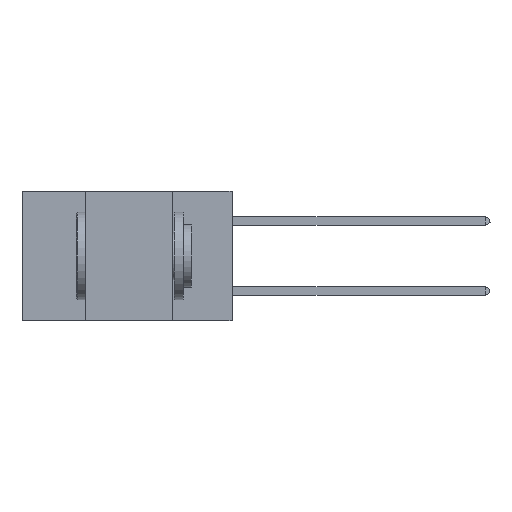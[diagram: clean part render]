
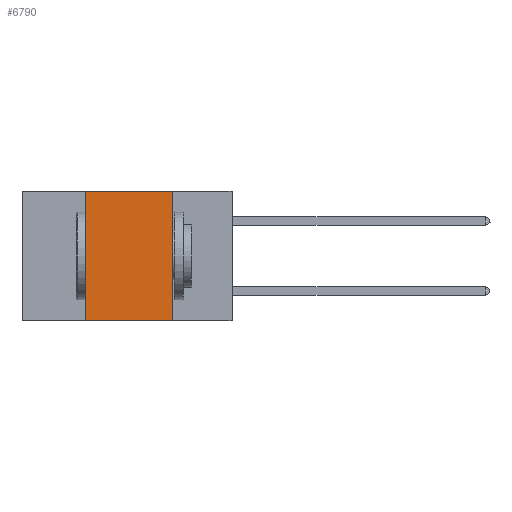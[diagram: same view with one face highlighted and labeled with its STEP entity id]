
A CAD part, left-side view. The second image highlights one B-rep face of the part: STEP entity #6790.
In plain terms, the highlighted planar face has unit normal (-1, 0, 0).
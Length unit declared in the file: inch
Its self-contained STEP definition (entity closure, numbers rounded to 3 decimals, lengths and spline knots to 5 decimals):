
#11 = DIRECTION ( 'NONE',  ( 0., -1., 0. ) ) ;
#507 = ORIENTED_EDGE ( 'NONE', *, *, #2817, .T. ) ;
#767 = CARTESIAN_POINT ( 'NONE',  ( 0., 0.6, 0. ) ) ;
#942 = VECTOR ( 'NONE', #11, 39.37008 ) ;
#2387 = CARTESIAN_POINT ( 'NONE',  ( 0., 0.6, 0. ) ) ;
#2694 = VERTEX_POINT ( 'NONE', #7048 ) ;
#2817 = EDGE_CURVE ( 'NONE', #7600, #11250, #10551, .T. ) ;
#3589 = CARTESIAN_POINT ( 'NONE',  ( 0., 0.6, -0.37 ) ) ;
#4266 = EDGE_CURVE ( 'NONE', #2694, #7081, #11045, .T. ) ;
#4537 = LINE ( 'NONE', #8906, #6108 ) ;
#4671 = EDGE_LOOP ( 'NONE', ( #9125, #9082, #5598, #507 ) ) ;
#4941 = LINE ( 'NONE', #5986, #10848 ) ;
#5598 = ORIENTED_EDGE ( 'NONE', *, *, #10435, .F. ) ;
#5986 = CARTESIAN_POINT ( 'NONE',  ( 0., 0.42, 0. ) ) ;
#6108 = VECTOR ( 'NONE', #8002, 39.37008 ) ;
#6155 = DIRECTION ( 'NONE',  ( 0., -1., 0. ) ) ;
#6216 = PLANE ( 'NONE',  #10685 ) ;
#6446 = CARTESIAN_POINT ( 'NONE',  ( 0., 0.17, 0. ) ) ;
#6533 = EDGE_CURVE ( 'NONE', #7081, #11250, #4537, .T. ) ;
#6790 = ADVANCED_FACE ( 'NONE', ( #10451 ), #6216, .F. ) ;
#7048 = CARTESIAN_POINT ( 'NONE',  ( 0., 0.42, 0. ) ) ;
#7081 = VERTEX_POINT ( 'NONE', #6446 ) ;
#7139 = DIRECTION ( 'NONE',  ( 1., 0., 0. ) ) ;
#7442 = VECTOR ( 'NONE', #6155, 39.37008 ) ;
#7600 = VERTEX_POINT ( 'NONE', #11287 ) ;
#8002 = DIRECTION ( 'NONE',  ( 0., 0., -1. ) ) ;
#8051 = DIRECTION ( 'NONE',  ( 0., 0., -1. ) ) ;
#8906 = CARTESIAN_POINT ( 'NONE',  ( 0., 0.17, 0. ) ) ;
#9082 = ORIENTED_EDGE ( 'NONE', *, *, #4266, .F. ) ;
#9125 = ORIENTED_EDGE ( 'NONE', *, *, #6533, .F. ) ;
#9638 = CARTESIAN_POINT ( 'NONE',  ( 0., 0.17, -0.37 ) ) ;
#10435 = EDGE_CURVE ( 'NONE', #7600, #2694, #4941, .T. ) ;
#10451 = FACE_OUTER_BOUND ( 'NONE', #4671, .T. ) ;
#10492 = DIRECTION ( 'NONE',  ( 0., 0., 1. ) ) ;
#10551 = LINE ( 'NONE', #3589, #942 ) ;
#10685 = AXIS2_PLACEMENT_3D ( 'NONE', #767, #7139, #8051 ) ;
#10848 = VECTOR ( 'NONE', #10492, 39.37008 ) ;
#11045 = LINE ( 'NONE', #2387, #7442 ) ;
#11250 = VERTEX_POINT ( 'NONE', #9638 ) ;
#11287 = CARTESIAN_POINT ( 'NONE',  ( 0., 0.42, -0.37 ) ) ;
